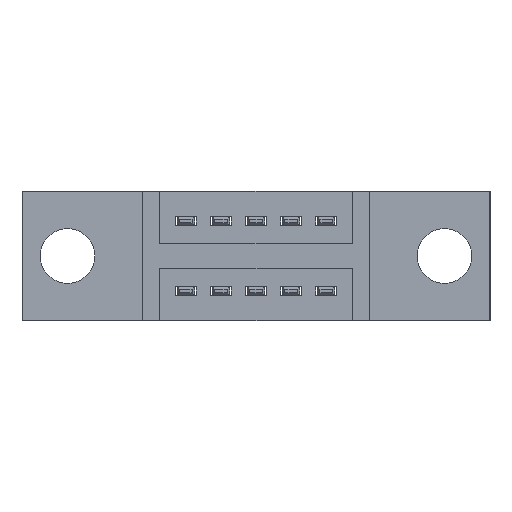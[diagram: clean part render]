
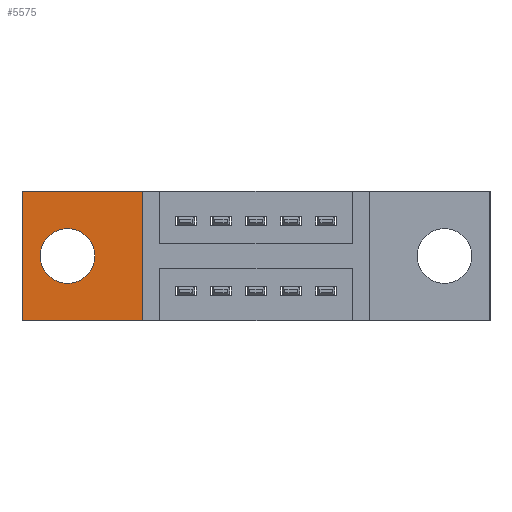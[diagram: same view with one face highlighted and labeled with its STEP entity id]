
A CAD part, front view. The second image highlights one B-rep face of the part: STEP entity #5575.
In plain terms, the highlighted planar face has unit normal (0, -1, 0).
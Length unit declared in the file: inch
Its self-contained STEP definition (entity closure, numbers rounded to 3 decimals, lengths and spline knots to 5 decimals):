
#22 = EDGE_CURVE ( 'NONE', #4070, #1307, #8101, .T. ) ;
#229 = DIRECTION ( 'NONE',  ( 0., -1., 0. ) ) ;
#350 = CARTESIAN_POINT ( 'NONE',  ( 0.3425, 0.11, 0. ) ) ;
#990 = DIRECTION ( 'NONE',  ( 0., 0., -1. ) ) ;
#1133 = CARTESIAN_POINT ( 'NONE',  ( 0.13, 0.11, -0.185 ) ) ;
#1307 = VERTEX_POINT ( 'NONE', #3369 ) ;
#1346 = DIRECTION ( 'NONE',  ( -1., 0., 0. ) ) ;
#1381 = VERTEX_POINT ( 'NONE', #5568 ) ;
#1669 = CARTESIAN_POINT ( 'NONE',  ( 0.3425, 0.11, -0.37 ) ) ;
#1819 = DIRECTION ( 'NONE',  ( 0., 0., -1. ) ) ;
#1831 = ORIENTED_EDGE ( 'NONE', *, *, #8233, .F. ) ;
#1890 = CARTESIAN_POINT ( 'NONE',  ( 0., 0.11, 0. ) ) ;
#2046 = ORIENTED_EDGE ( 'NONE', *, *, #4655, .T. ) ;
#2241 = CARTESIAN_POINT ( 'NONE',  ( 0., 0.11, -0.37 ) ) ;
#2420 = DIRECTION ( 'NONE',  ( 0., 0., 1. ) ) ;
#2452 = EDGE_CURVE ( 'NONE', #7669, #3696, #8066, .T. ) ;
#2628 = DIRECTION ( 'NONE',  ( 0., 0., -1. ) ) ;
#2667 = LINE ( 'NONE', #5444, #6121 ) ;
#2943 = VECTOR ( 'NONE', #990, 39.37008 ) ;
#3010 = CARTESIAN_POINT ( 'NONE',  ( 0.13, 0.11, -0.263 ) ) ;
#3085 = AXIS2_PLACEMENT_3D ( 'NONE', #5991, #5517, #2628 ) ;
#3200 = CARTESIAN_POINT ( 'NONE',  ( 0.13, 0.11, -0.185 ) ) ;
#3233 = FACE_BOUND ( 'NONE', #6542, .T. ) ;
#3334 = LINE ( 'NONE', #2241, #4964 ) ;
#3369 = CARTESIAN_POINT ( 'NONE',  ( 0.3425, 0.11, 0. ) ) ;
#3433 = PLANE ( 'NONE',  #3085 ) ;
#3461 = VERTEX_POINT ( 'NONE', #4092 ) ;
#3696 = VERTEX_POINT ( 'NONE', #3736 ) ;
#3736 = CARTESIAN_POINT ( 'NONE',  ( 0.13, 0.11, -0.107 ) ) ;
#3846 = ORIENTED_EDGE ( 'NONE', *, *, #6191, .T. ) ;
#4070 = VERTEX_POINT ( 'NONE', #1669 ) ;
#4092 = CARTESIAN_POINT ( 'NONE',  ( 0., 0.11, -0.37 ) ) ;
#4159 = AXIS2_PLACEMENT_3D ( 'NONE', #1133, #5912, #1819 ) ;
#4655 = EDGE_CURVE ( 'NONE', #1381, #3461, #4764, .T. ) ;
#4764 = LINE ( 'NONE', #1890, #2943 ) ;
#4891 = EDGE_LOOP ( 'NONE', ( #2046, #3846, #5679, #7702 ) ) ;
#4964 = VECTOR ( 'NONE', #7020, 39.37008 ) ;
#5444 = CARTESIAN_POINT ( 'NONE',  ( 0., 0.11, 0. ) ) ;
#5468 = ORIENTED_EDGE ( 'NONE', *, *, #2452, .F. ) ;
#5517 = DIRECTION ( 'NONE',  ( 0., -1., 0. ) ) ;
#5568 = CARTESIAN_POINT ( 'NONE',  ( 0., 0.11, 0. ) ) ;
#5575 = ADVANCED_FACE ( 'NONE', ( #3233, #6913 ), #3433, .T. ) ;
#5679 = ORIENTED_EDGE ( 'NONE', *, *, #22, .T. ) ;
#5688 = CIRCLE ( 'NONE', #4159, 0.078 ) ;
#5912 = DIRECTION ( 'NONE',  ( 0., -1., 0. ) ) ;
#5991 = CARTESIAN_POINT ( 'NONE',  ( 0., 0.11, -0.37 ) ) ;
#6121 = VECTOR ( 'NONE', #1346, 39.37008 ) ;
#6191 = EDGE_CURVE ( 'NONE', #3461, #4070, #3334, .T. ) ;
#6320 = VECTOR ( 'NONE', #2420, 39.37008 ) ;
#6542 = EDGE_LOOP ( 'NONE', ( #1831, #5468 ) ) ;
#6913 = FACE_OUTER_BOUND ( 'NONE', #4891, .T. ) ;
#7020 = DIRECTION ( 'NONE',  ( 1., 0., 0. ) ) ;
#7669 = VERTEX_POINT ( 'NONE', #3010 ) ;
#7702 = ORIENTED_EDGE ( 'NONE', *, *, #7938, .T. ) ;
#7906 = DIRECTION ( 'NONE',  ( 0., 0., -1. ) ) ;
#7938 = EDGE_CURVE ( 'NONE', #1307, #1381, #2667, .T. ) ;
#8066 = CIRCLE ( 'NONE', #8167, 0.078 ) ;
#8101 = LINE ( 'NONE', #350, #6320 ) ;
#8167 = AXIS2_PLACEMENT_3D ( 'NONE', #3200, #229, #7906 ) ;
#8233 = EDGE_CURVE ( 'NONE', #3696, #7669, #5688, .T. ) ;
